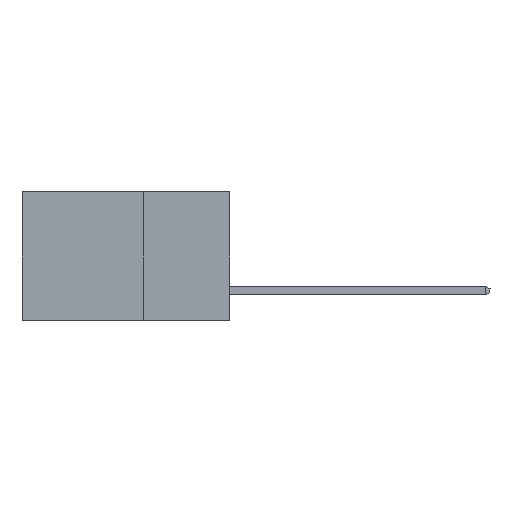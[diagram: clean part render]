
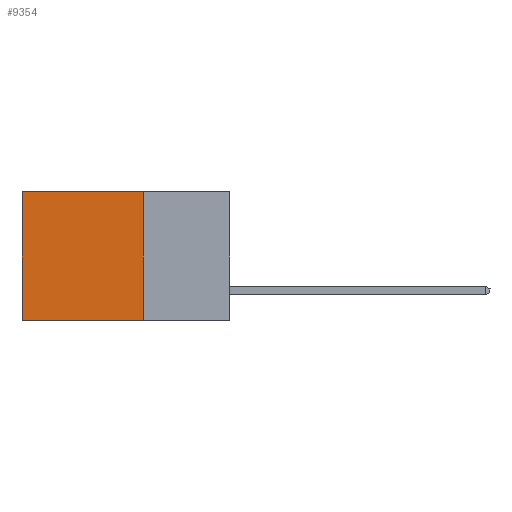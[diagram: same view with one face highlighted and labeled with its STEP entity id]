
A CAD part, left-side view. The second image highlights one B-rep face of the part: STEP entity #9354.
In plain terms, the highlighted planar face has unit normal (-1, 0, 0).
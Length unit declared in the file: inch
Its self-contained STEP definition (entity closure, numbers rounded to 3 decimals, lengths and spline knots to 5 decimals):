
#21 = CARTESIAN_POINT ( 'NONE',  ( 0.2615, 0.25, -0.37 ) ) ;
#38 = CARTESIAN_POINT ( 'NONE',  ( 0.2615, 0.25, -0.37 ) ) ;
#52 = ORIENTED_EDGE ( 'NONE', *, *, #7146, .T. ) ;
#433 = CARTESIAN_POINT ( 'NONE',  ( 0.2615, 0.25, -0.37 ) ) ;
#517 = VECTOR ( 'NONE', #13024, 39.37008 ) ;
#971 = VECTOR ( 'NONE', #11810, 39.37008 ) ;
#1930 = DIRECTION ( 'NONE',  ( 0., 0., -1. ) ) ;
#3856 = FACE_OUTER_BOUND ( 'NONE', #7473, .T. ) ;
#4014 = CARTESIAN_POINT ( 'NONE',  ( 0.2615, 0.6, 0. ) ) ;
#4299 = AXIS2_PLACEMENT_3D ( 'NONE', #38, #13040, #1930 ) ;
#4508 = ORIENTED_EDGE ( 'NONE', *, *, #15826, .T. ) ;
#5297 = ORIENTED_EDGE ( 'NONE', *, *, #19751, .F. ) ;
#6067 = VERTEX_POINT ( 'NONE', #433 ) ;
#6495 = VERTEX_POINT ( 'NONE', #15914 ) ;
#6872 = DIRECTION ( 'NONE',  ( 0., 1., 0. ) ) ;
#7146 = EDGE_CURVE ( 'NONE', #6495, #13501, #9489, .T. ) ;
#7473 = EDGE_LOOP ( 'NONE', ( #4508, #18872, #5297, #52 ) ) ;
#7835 = CARTESIAN_POINT ( 'NONE',  ( 0.2615, 0.25, 0. ) ) ;
#8446 = CARTESIAN_POINT ( 'NONE',  ( 0.2615, 0.6, -0.37 ) ) ;
#9354 = ADVANCED_FACE ( 'NONE', ( #3856 ), #14765, .F. ) ;
#9489 = LINE ( 'NONE', #7835, #13775 ) ;
#11730 = VERTEX_POINT ( 'NONE', #8446 ) ;
#11810 = DIRECTION ( 'NONE',  ( 0., 0., -1. ) ) ;
#12020 = CARTESIAN_POINT ( 'NONE',  ( 0.2615, 0.6, -0.37 ) ) ;
#13024 = DIRECTION ( 'NONE',  ( 0., 1., 0. ) ) ;
#13040 = DIRECTION ( 'NONE',  ( 1., 0., 0. ) ) ;
#13501 = VERTEX_POINT ( 'NONE', #4014 ) ;
#13582 = LINE ( 'NONE', #12020, #22252 ) ;
#13775 = VECTOR ( 'NONE', #6872, 39.37008 ) ;
#14765 = PLANE ( 'NONE',  #4299 ) ;
#15826 = EDGE_CURVE ( 'NONE', #13501, #11730, #13582, .T. ) ;
#15914 = CARTESIAN_POINT ( 'NONE',  ( 0.2615, 0.25, 0. ) ) ;
#16186 = EDGE_CURVE ( 'NONE', #6067, #11730, #18780, .T. ) ;
#17353 = DIRECTION ( 'NONE',  ( 0., 0., -1. ) ) ;
#18780 = LINE ( 'NONE', #21, #517 ) ;
#18872 = ORIENTED_EDGE ( 'NONE', *, *, #16186, .F. ) ;
#19751 = EDGE_CURVE ( 'NONE', #6495, #6067, #20249, .T. ) ;
#20249 = LINE ( 'NONE', #20524, #971 ) ;
#20524 = CARTESIAN_POINT ( 'NONE',  ( 0.2615, 0.25, -0.37 ) ) ;
#22252 = VECTOR ( 'NONE', #17353, 39.37008 ) ;
